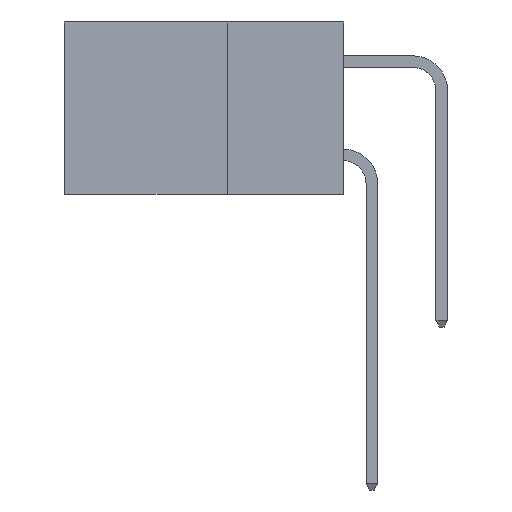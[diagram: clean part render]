
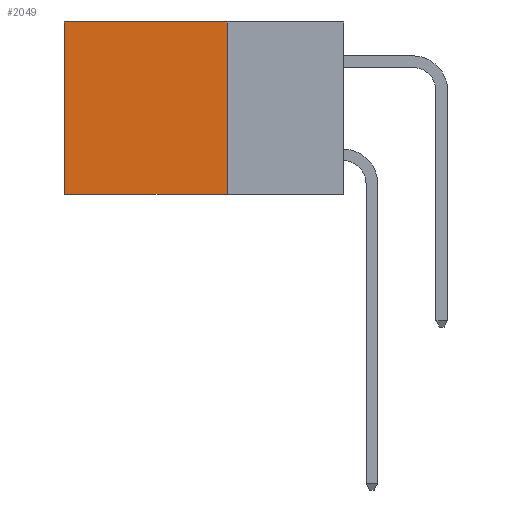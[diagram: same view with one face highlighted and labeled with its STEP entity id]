
A CAD part, left-side view. The second image highlights one B-rep face of the part: STEP entity #2049.
In plain terms, the highlighted planar face has unit normal (-1, 0, 0).
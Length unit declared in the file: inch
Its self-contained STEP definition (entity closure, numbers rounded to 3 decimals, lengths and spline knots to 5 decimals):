
#414 = DIRECTION ( 'NONE',  ( 0., 0., -1. ) ) ;
#665 = EDGE_LOOP ( 'NONE', ( #18360, #11167, #12482, #17694 ) ) ;
#1442 = VECTOR ( 'NONE', #12817, 39.37008 ) ;
#1456 = VERTEX_POINT ( 'NONE', #10320 ) ;
#2049 = ADVANCED_FACE ( 'NONE', ( #20336 ), #18024, .F. ) ;
#2138 = DIRECTION ( 'NONE',  ( 0., 0., -1. ) ) ;
#2492 = VERTEX_POINT ( 'NONE', #11527 ) ;
#3903 = EDGE_CURVE ( 'NONE', #2492, #1456, #7076, .T. ) ;
#4162 = EDGE_CURVE ( 'NONE', #9335, #2492, #20280, .T. ) ;
#5447 = LINE ( 'NONE', #17783, #1442 ) ;
#7076 = LINE ( 'NONE', #20520, #11530 ) ;
#8332 = DIRECTION ( 'NONE',  ( 0., 1., 0. ) ) ;
#9335 = VERTEX_POINT ( 'NONE', #18054 ) ;
#9568 = CARTESIAN_POINT ( 'NONE',  ( 0.2615, 0.25, 0. ) ) ;
#10022 = CARTESIAN_POINT ( 'NONE',  ( 0.2615, 0.25, -0.37 ) ) ;
#10320 = CARTESIAN_POINT ( 'NONE',  ( 0.2615, 0.6, -0.37 ) ) ;
#10825 = LINE ( 'NONE', #10022, #14721 ) ;
#11167 = ORIENTED_EDGE ( 'NONE', *, *, #12144, .F. ) ;
#11197 = CARTESIAN_POINT ( 'NONE',  ( 0.2615, 0.25, -0.37 ) ) ;
#11250 = DIRECTION ( 'NONE',  ( 0., 1., 0. ) ) ;
#11527 = CARTESIAN_POINT ( 'NONE',  ( 0.2615, 0.6, 0. ) ) ;
#11530 = VECTOR ( 'NONE', #414, 39.37008 ) ;
#11554 = VECTOR ( 'NONE', #11250, 39.37008 ) ;
#11930 = VERTEX_POINT ( 'NONE', #11197 ) ;
#12144 = EDGE_CURVE ( 'NONE', #11930, #1456, #10825, .T. ) ;
#12482 = ORIENTED_EDGE ( 'NONE', *, *, #15009, .F. ) ;
#12817 = DIRECTION ( 'NONE',  ( 0., 0., -1. ) ) ;
#14721 = VECTOR ( 'NONE', #8332, 39.37008 ) ;
#15009 = EDGE_CURVE ( 'NONE', #9335, #11930, #5447, .T. ) ;
#17694 = ORIENTED_EDGE ( 'NONE', *, *, #4162, .T. ) ;
#17783 = CARTESIAN_POINT ( 'NONE',  ( 0.2615, 0.25, -0.37 ) ) ;
#17815 = CARTESIAN_POINT ( 'NONE',  ( 0.2615, 0.25, -0.37 ) ) ;
#18024 = PLANE ( 'NONE',  #20561 ) ;
#18054 = CARTESIAN_POINT ( 'NONE',  ( 0.2615, 0.25, 0. ) ) ;
#18235 = DIRECTION ( 'NONE',  ( 1., 0., 0. ) ) ;
#18360 = ORIENTED_EDGE ( 'NONE', *, *, #3903, .T. ) ;
#20280 = LINE ( 'NONE', #9568, #11554 ) ;
#20336 = FACE_OUTER_BOUND ( 'NONE', #665, .T. ) ;
#20520 = CARTESIAN_POINT ( 'NONE',  ( 0.2615, 0.6, -0.37 ) ) ;
#20561 = AXIS2_PLACEMENT_3D ( 'NONE', #17815, #18235, #2138 ) ;
